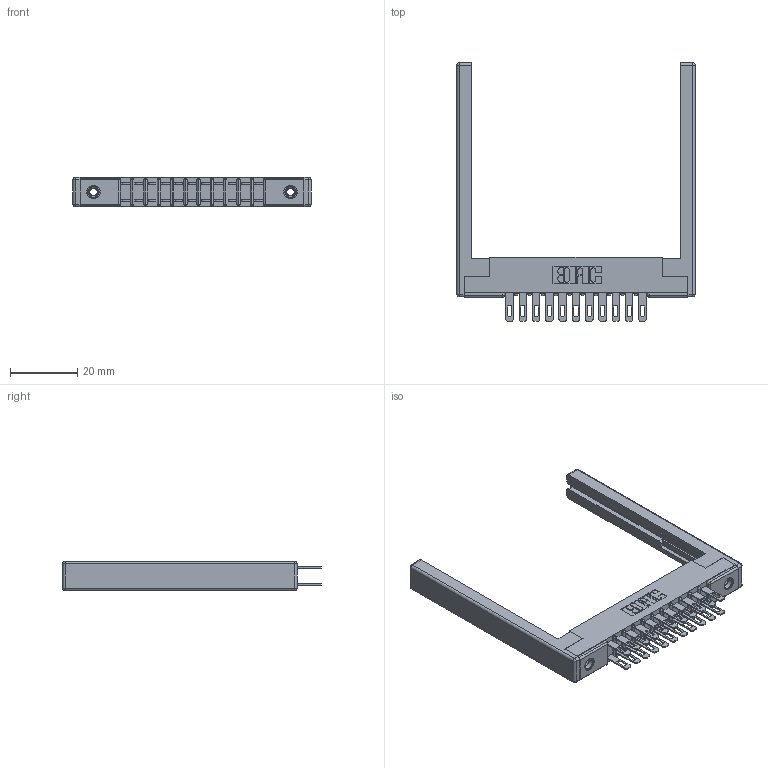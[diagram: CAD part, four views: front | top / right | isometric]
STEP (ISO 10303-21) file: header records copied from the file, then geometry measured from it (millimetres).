
FILE_DESCRIPTION (( 'STEP AP203' ), '1' );
FILE_NAME ('307-022-500-268.STEP', '2019-09-05T21:08:35', ( '' ), ( '' ), 'SwSTEP 2.0', 'SolidWorks 2016', '' );
FILE_SCHEMA (( 'CONFIG_CONTROL_DESIGN' ));
Length unit declared in the file: inch
Products named in the file (5): 307-290-001_500; 345-250-001_345-250-001-102; 307-022-500-268; 307 Part_.156 Dia Mounting Holes; 307-220-068
Assembly tree (27 placements, depth 2):
  307-022-500-268
    307 Part_.156 Dia Mounting Holes
    307-290-001_500  x22
    307-220-068  x2
    345-250-001_345-250-001-102  x2
Bounding box: 71.02 x 77.14 x 8.71 mm (x, y, z)
Volume: 9271.1 mm3; surface area: 12138.3 mm2
Topology: 27 solids, 27 shells, 1296 faces, 3573 edges, 2298 vertices
Faces by surface type: plane 818, cylinder 430, sphere 32, cone 12, torus 4
Entity records: 16337 total; most frequent: CARTESIAN_POINT 2656, DIRECTION 2632, ORIENTED_EDGE 2620, EDGE_CURVE 1310, VECTOR 988, LINE 988, VERTEX_POINT 846, AXIS2_PLACEMENT_3D 822
